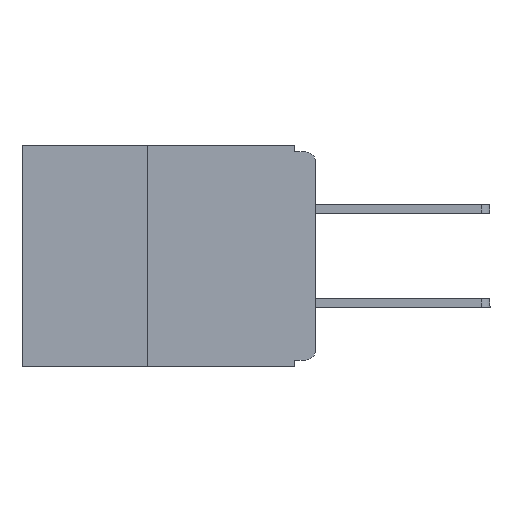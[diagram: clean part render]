
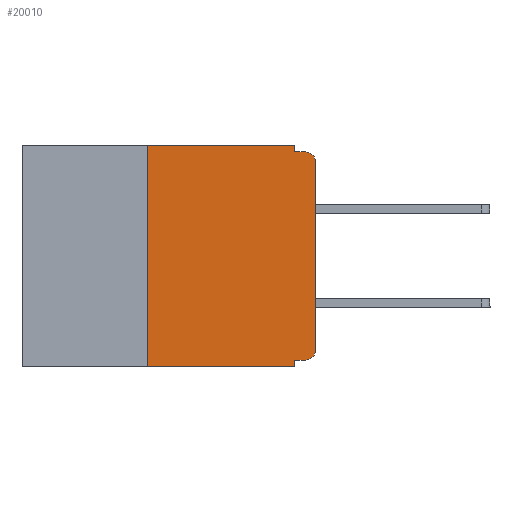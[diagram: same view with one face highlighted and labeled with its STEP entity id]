
A CAD part, left-side view. The second image highlights one B-rep face of the part: STEP entity #20010.
In plain terms, the highlighted planar face has unit normal (-1, 0, 0).
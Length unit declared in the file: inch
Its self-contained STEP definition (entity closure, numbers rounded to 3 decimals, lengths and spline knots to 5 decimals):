
#852 = VERTEX_POINT ( 'NONE', #23820 ) ;
#1172 = AXIS2_PLACEMENT_3D ( 'NONE', #32147, #17394, #2183 ) ;
#1886 = LINE ( 'NONE', #29817, #8758 ) ;
#2086 = VERTEX_POINT ( 'NONE', #16916 ) ;
#2183 = DIRECTION ( 'NONE',  ( 0., 0., -1. ) ) ;
#2347 = CARTESIAN_POINT ( 'NONE',  ( 0., 0.015, -0.32 ) ) ;
#2665 = CARTESIAN_POINT ( 'NONE',  ( 0., 0.031, -0.33 ) ) ;
#2916 = VERTEX_POINT ( 'NONE', #2347 ) ;
#3222 = VERTEX_POINT ( 'NONE', #2665 ) ;
#3258 = ORIENTED_EDGE ( 'NONE', *, *, #21188, .F. ) ;
#3494 = LINE ( 'NONE', #10106, #28615 ) ;
#3715 = VERTEX_POINT ( 'NONE', #11322 ) ;
#4458 = EDGE_CURVE ( 'NONE', #3715, #12518, #29055, .T. ) ;
#4517 = LINE ( 'NONE', #32241, #30293 ) ;
#4790 = EDGE_CURVE ( 'NONE', #2086, #3715, #1886, .T. ) ;
#4870 = CARTESIAN_POINT ( 'NONE',  ( 0., 0.031, 0. ) ) ;
#4904 = VERTEX_POINT ( 'NONE', #23005 ) ;
#4912 = DIRECTION ( 'NONE',  ( 0., 0., -1. ) ) ;
#5142 = EDGE_CURVE ( 'NONE', #2916, #852, #3494, .T. ) ;
#6653 = CARTESIAN_POINT ( 'NONE',  ( 0., 0., -0.01 ) ) ;
#6666 = EDGE_CURVE ( 'NONE', #22167, #7809, #18069, .T. ) ;
#6930 = DIRECTION ( 'NONE',  ( 0., 0., -1. ) ) ;
#7303 = EDGE_CURVE ( 'NONE', #7809, #4904, #12537, .T. ) ;
#7751 = AXIS2_PLACEMENT_3D ( 'NONE', #9244, #21977, #6930 ) ;
#7809 = VERTEX_POINT ( 'NONE', #14395 ) ;
#7978 = EDGE_CURVE ( 'NONE', #23740, #22167, #4517, .T. ) ;
#8373 = CARTESIAN_POINT ( 'NONE',  ( 0., 0.25, 0. ) ) ;
#8758 = VECTOR ( 'NONE', #29480, 39.37008 ) ;
#9244 = CARTESIAN_POINT ( 'NONE',  ( 0., 0.437, 0. ) ) ;
#10106 = CARTESIAN_POINT ( 'NONE',  ( 0., 0., -0.32 ) ) ;
#10849 = ORIENTED_EDGE ( 'NONE', *, *, #5142, .F. ) ;
#10875 = ORIENTED_EDGE ( 'NONE', *, *, #16007, .T. ) ;
#11043 = CARTESIAN_POINT ( 'NONE',  ( 0., 0.25, -0.33 ) ) ;
#11322 = CARTESIAN_POINT ( 'NONE',  ( 0., 0., -0.025 ) ) ;
#11330 = AXIS2_PLACEMENT_3D ( 'NONE', #14635, #15223, #15175 ) ;
#12452 = VECTOR ( 'NONE', #25842, 39.37008 ) ;
#12518 = VERTEX_POINT ( 'NONE', #20780 ) ;
#12537 = LINE ( 'NONE', #4870, #18425 ) ;
#12977 = VECTOR ( 'NONE', #14788, 39.37008 ) ;
#13891 = FACE_OUTER_BOUND ( 'NONE', #29356, .T. ) ;
#14395 = CARTESIAN_POINT ( 'NONE',  ( 0., 0.031, 0. ) ) ;
#14635 = CARTESIAN_POINT ( 'NONE',  ( 0., 0.015, -0.025 ) ) ;
#14751 = DIRECTION ( 'NONE',  ( 0., 1., 0. ) ) ;
#14788 = DIRECTION ( 'NONE',  ( 0., -1., 0. ) ) ;
#14794 = CARTESIAN_POINT ( 'NONE',  ( 0., 0.437, 0. ) ) ;
#15039 = ORIENTED_EDGE ( 'NONE', *, *, #6666, .F. ) ;
#15175 = DIRECTION ( 'NONE',  ( 0., 0., -1. ) ) ;
#15223 = DIRECTION ( 'NONE',  ( -1., 0., 0. ) ) ;
#15270 = ORIENTED_EDGE ( 'NONE', *, *, #7303, .F. ) ;
#15429 = EDGE_CURVE ( 'NONE', #23740, #3222, #25139, .T. ) ;
#16007 = EDGE_CURVE ( 'NONE', #2916, #2086, #27394, .T. ) ;
#16913 = ORIENTED_EDGE ( 'NONE', *, *, #4458, .T. ) ;
#16916 = CARTESIAN_POINT ( 'NONE',  ( 0., 0., -0.305 ) ) ;
#16948 = ORIENTED_EDGE ( 'NONE', *, *, #4790, .T. ) ;
#17394 = DIRECTION ( 'NONE',  ( -1., 0., 0. ) ) ;
#17721 = VECTOR ( 'NONE', #21691, 39.37008 ) ;
#18069 = LINE ( 'NONE', #14794, #12977 ) ;
#18256 = ORIENTED_EDGE ( 'NONE', *, *, #22771, .F. ) ;
#18425 = VECTOR ( 'NONE', #4912, 39.37008 ) ;
#18912 = ORIENTED_EDGE ( 'NONE', *, *, #15429, .T. ) ;
#18939 = ORIENTED_EDGE ( 'NONE', *, *, #7978, .F. ) ;
#20010 = ADVANCED_FACE ( 'NONE', ( #13891 ), #29274, .F. ) ;
#20070 = DIRECTION ( 'NONE',  ( 0., -1., 0. ) ) ;
#20780 = CARTESIAN_POINT ( 'NONE',  ( 0., 0.015, -0.01 ) ) ;
#21188 = EDGE_CURVE ( 'NONE', #4904, #12518, #30826, .T. ) ;
#21691 = DIRECTION ( 'NONE',  ( 0., -1., 0. ) ) ;
#21977 = DIRECTION ( 'NONE',  ( 1., 0., 0. ) ) ;
#22167 = VERTEX_POINT ( 'NONE', #8373 ) ;
#22575 = CARTESIAN_POINT ( 'NONE',  ( 0., 0.437, -0.33 ) ) ;
#22771 = EDGE_CURVE ( 'NONE', #852, #3222, #32171, .T. ) ;
#23005 = CARTESIAN_POINT ( 'NONE',  ( 0., 0.031, -0.01 ) ) ;
#23341 = CARTESIAN_POINT ( 'NONE',  ( 0., 0.031, -0.33 ) ) ;
#23740 = VERTEX_POINT ( 'NONE', #11043 ) ;
#23820 = CARTESIAN_POINT ( 'NONE',  ( 0., 0.031, -0.32 ) ) ;
#24341 = VECTOR ( 'NONE', #20070, 39.37008 ) ;
#25139 = LINE ( 'NONE', #22575, #24341 ) ;
#25842 = DIRECTION ( 'NONE',  ( 0., 0., -1. ) ) ;
#27394 = CIRCLE ( 'NONE', #1172, 0.015 ) ;
#28615 = VECTOR ( 'NONE', #14751, 39.37008 ) ;
#29055 = CIRCLE ( 'NONE', #11330, 0.015 ) ;
#29274 = PLANE ( 'NONE',  #7751 ) ;
#29356 = EDGE_LOOP ( 'NONE', ( #16948, #16913, #3258, #15270, #15039, #18939, #18912, #18256, #10849, #10875 ) ) ;
#29480 = DIRECTION ( 'NONE',  ( 0., 0., 1. ) ) ;
#29817 = CARTESIAN_POINT ( 'NONE',  ( 0., 0., 0. ) ) ;
#30293 = VECTOR ( 'NONE', #32132, 39.37008 ) ;
#30826 = LINE ( 'NONE', #6653, #17721 ) ;
#32132 = DIRECTION ( 'NONE',  ( 0., 0., 1. ) ) ;
#32147 = CARTESIAN_POINT ( 'NONE',  ( 0., 0.015, -0.305 ) ) ;
#32171 = LINE ( 'NONE', #23341, #12452 ) ;
#32241 = CARTESIAN_POINT ( 'NONE',  ( 0., 0.25, -0.33 ) ) ;
